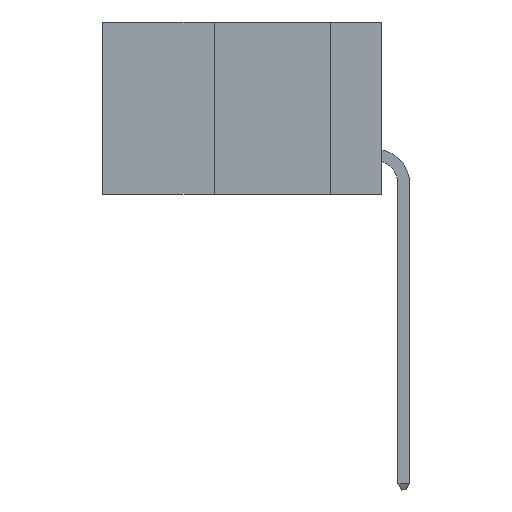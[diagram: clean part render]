
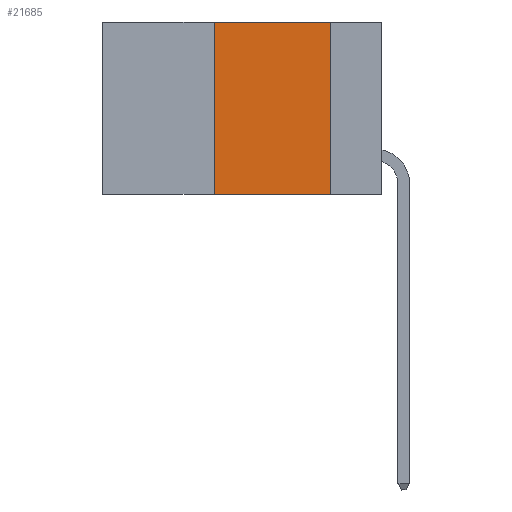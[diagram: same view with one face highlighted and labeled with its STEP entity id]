
A CAD part, left-side view. The second image highlights one B-rep face of the part: STEP entity #21685.
In plain terms, the highlighted planar face has unit normal (-1, 0, 0).
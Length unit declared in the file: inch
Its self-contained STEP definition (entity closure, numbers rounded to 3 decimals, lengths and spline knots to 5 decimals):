
#97 = VERTEX_POINT ( 'NONE', #20087 ) ;
#554 = EDGE_CURVE ( 'NONE', #25096, #7057, #10234, .T. ) ;
#619 = VECTOR ( 'NONE', #6591, 39.37008 ) ;
#2225 = EDGE_LOOP ( 'NONE', ( #23765, #4048, #6661, #16186 ) ) ;
#3194 = CARTESIAN_POINT ( 'NONE',  ( 0., 0.6, 0. ) ) ;
#4048 = ORIENTED_EDGE ( 'NONE', *, *, #9999, .F. ) ;
#4852 = LINE ( 'NONE', #7219, #15564 ) ;
#6060 = VERTEX_POINT ( 'NONE', #15261 ) ;
#6498 = CARTESIAN_POINT ( 'NONE',  ( 0., 0.6, -0.37 ) ) ;
#6591 = DIRECTION ( 'NONE',  ( 0., -1., 0. ) ) ;
#6661 = ORIENTED_EDGE ( 'NONE', *, *, #554, .F. ) ;
#7057 = VERTEX_POINT ( 'NONE', #14066 ) ;
#7219 = CARTESIAN_POINT ( 'NONE',  ( 0., 0.6, 0. ) ) ;
#7780 = CARTESIAN_POINT ( 'NONE',  ( 0., 0.36, 0. ) ) ;
#9999 = EDGE_CURVE ( 'NONE', #7057, #97, #4852, .T. ) ;
#10234 = LINE ( 'NONE', #7780, #25769 ) ;
#11457 = DIRECTION ( 'NONE',  ( 0., -1., 0. ) ) ;
#13840 = LINE ( 'NONE', #21817, #19023 ) ;
#14066 = CARTESIAN_POINT ( 'NONE',  ( 0., 0.36, 0. ) ) ;
#14908 = AXIS2_PLACEMENT_3D ( 'NONE', #3194, #26291, #20119 ) ;
#15261 = CARTESIAN_POINT ( 'NONE',  ( 0., 0.11, -0.37 ) ) ;
#15564 = VECTOR ( 'NONE', #11457, 39.37008 ) ;
#15687 = DIRECTION ( 'NONE',  ( 0., 0., 1. ) ) ;
#16186 = ORIENTED_EDGE ( 'NONE', *, *, #16584, .T. ) ;
#16584 = EDGE_CURVE ( 'NONE', #25096, #6060, #24955, .T. ) ;
#18068 = PLANE ( 'NONE',  #14908 ) ;
#19023 = VECTOR ( 'NONE', #23907, 39.37008 ) ;
#20087 = CARTESIAN_POINT ( 'NONE',  ( 0., 0.11, 0. ) ) ;
#20119 = DIRECTION ( 'NONE',  ( 0., 0., -1. ) ) ;
#20734 = CARTESIAN_POINT ( 'NONE',  ( 0., 0.36, -0.37 ) ) ;
#21035 = EDGE_CURVE ( 'NONE', #97, #6060, #13840, .T. ) ;
#21685 = ADVANCED_FACE ( 'NONE', ( #23527 ), #18068, .F. ) ;
#21817 = CARTESIAN_POINT ( 'NONE',  ( 0., 0.11, 0. ) ) ;
#23527 = FACE_OUTER_BOUND ( 'NONE', #2225, .T. ) ;
#23765 = ORIENTED_EDGE ( 'NONE', *, *, #21035, .F. ) ;
#23907 = DIRECTION ( 'NONE',  ( 0., 0., -1. ) ) ;
#24955 = LINE ( 'NONE', #6498, #619 ) ;
#25096 = VERTEX_POINT ( 'NONE', #20734 ) ;
#25769 = VECTOR ( 'NONE', #15687, 39.37008 ) ;
#26291 = DIRECTION ( 'NONE',  ( 1., 0., 0. ) ) ;
